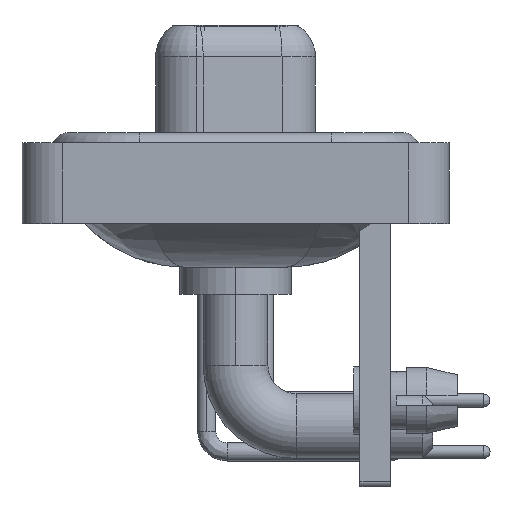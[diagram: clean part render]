
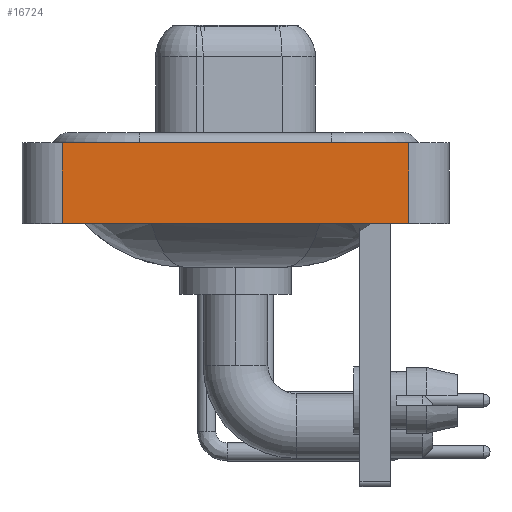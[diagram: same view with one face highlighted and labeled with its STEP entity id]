
A CAD part, left-side view. The second image highlights one B-rep face of the part: STEP entity #16724.
In plain terms, the highlighted planar face has unit normal (-1, 0, 0).
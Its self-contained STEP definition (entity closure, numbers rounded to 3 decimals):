
#647 = CARTESIAN_POINT ( 'NONE',  ( -7.35, 8.55, -3.6 ) ) ;
#1104 = DIRECTION ( 'NONE',  ( -1., 0., 0. ) ) ;
#1987 = VECTOR ( 'NONE', #22673, 1000. ) ;
#2005 = EDGE_CURVE ( 'NONE', #9301, #4445, #3154, .T. ) ;
#2252 = EDGE_CURVE ( 'NONE', #19576, #2548, #2429, .T. ) ;
#2429 = LINE ( 'NONE', #4217, #14095 ) ;
#2548 = VERTEX_POINT ( 'NONE', #5705 ) ;
#2803 = CARTESIAN_POINT ( 'NONE',  ( -7.35, 8.55, -3.6 ) ) ;
#3154 = LINE ( 'NONE', #2803, #14070 ) ;
#4217 = CARTESIAN_POINT ( 'NONE',  ( -7.35, -8.55, -3.6 ) ) ;
#4445 = VERTEX_POINT ( 'NONE', #5688 ) ;
#5688 = CARTESIAN_POINT ( 'NONE',  ( -7.35, 8.55, 0.4 ) ) ;
#5705 = CARTESIAN_POINT ( 'NONE',  ( -7.35, -8.55, 0.4 ) ) ;
#5760 = DIRECTION ( 'NONE',  ( 0., 0., 1. ) ) ;
#5800 = ORIENTED_EDGE ( 'NONE', *, *, #19531, .T. ) ;
#6033 = VECTOR ( 'NONE', #11269, 1000. ) ;
#6815 = FACE_OUTER_BOUND ( 'NONE', #13367, .T. ) ;
#7482 = LINE ( 'NONE', #12915, #6033 ) ;
#7999 = AXIS2_PLACEMENT_3D ( 'NONE', #21167, #1104, #8146 ) ;
#8146 = DIRECTION ( 'NONE',  ( 0., 0., 1. ) ) ;
#8364 = PLANE ( 'NONE',  #7999 ) ;
#9301 = VERTEX_POINT ( 'NONE', #647 ) ;
#10365 = CARTESIAN_POINT ( 'NONE',  ( -7.35, -8.55, -3.6 ) ) ;
#10424 = DIRECTION ( 'NONE',  ( 0., 0., 1. ) ) ;
#11269 = DIRECTION ( 'NONE',  ( 0., -1., 0. ) ) ;
#12915 = CARTESIAN_POINT ( 'NONE',  ( -7.35, -8.55, 0.4 ) ) ;
#13367 = EDGE_LOOP ( 'NONE', ( #20174, #15150, #15498, #5800 ) ) ;
#14070 = VECTOR ( 'NONE', #10424, 1000. ) ;
#14095 = VECTOR ( 'NONE', #5760, 1000. ) ;
#15150 = ORIENTED_EDGE ( 'NONE', *, *, #23208, .F. ) ;
#15498 = ORIENTED_EDGE ( 'NONE', *, *, #2005, .F. ) ;
#16154 = CARTESIAN_POINT ( 'NONE',  ( -7.35, -8.55, -3.6 ) ) ;
#16724 = ADVANCED_FACE ( 'NONE', ( #6815 ), #8364, .T. ) ;
#19531 = EDGE_CURVE ( 'NONE', #9301, #19576, #21133, .T. ) ;
#19576 = VERTEX_POINT ( 'NONE', #16154 ) ;
#20174 = ORIENTED_EDGE ( 'NONE', *, *, #2252, .T. ) ;
#21133 = LINE ( 'NONE', #10365, #1987 ) ;
#21167 = CARTESIAN_POINT ( 'NONE',  ( -7.35, -8.55, -3.6 ) ) ;
#22673 = DIRECTION ( 'NONE',  ( 0., -1., 0. ) ) ;
#23208 = EDGE_CURVE ( 'NONE', #4445, #2548, #7482, .T. ) ;
